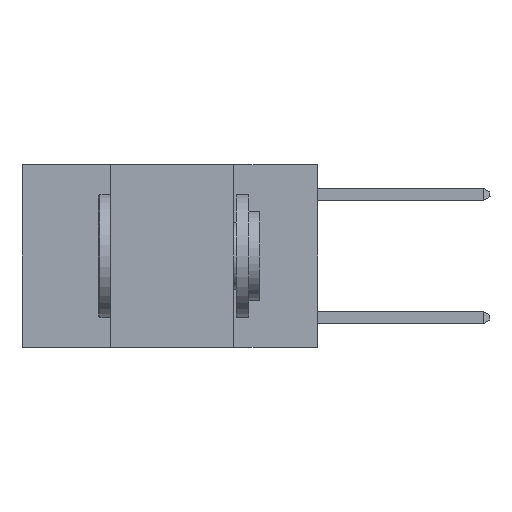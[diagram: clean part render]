
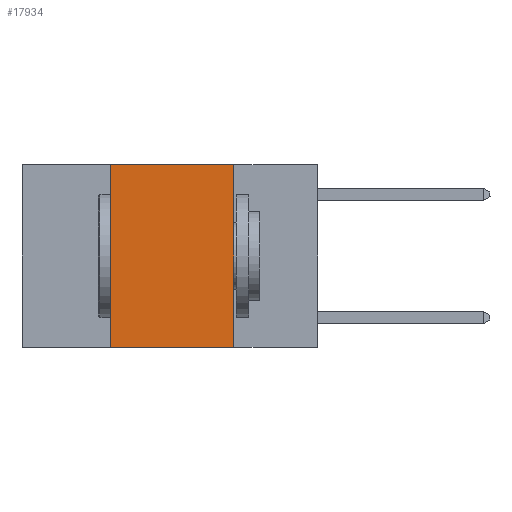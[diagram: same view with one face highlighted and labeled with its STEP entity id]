
A CAD part, left-side view. The second image highlights one B-rep face of the part: STEP entity #17934.
In plain terms, the highlighted planar face has unit normal (-1, 0, 0).
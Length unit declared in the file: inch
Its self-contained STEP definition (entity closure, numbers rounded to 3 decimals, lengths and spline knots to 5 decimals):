
#797 = ORIENTED_EDGE ( 'NONE', *, *, #24428, .T. ) ;
#1417 = VERTEX_POINT ( 'NONE', #14738 ) ;
#2218 = EDGE_CURVE ( 'NONE', #12033, #11483, #13702, .T. ) ;
#2584 = DIRECTION ( 'NONE',  ( 1., 0., 0. ) ) ;
#2837 = VECTOR ( 'NONE', #30920, 39.37008 ) ;
#5230 = VECTOR ( 'NONE', #6433, 39.37008 ) ;
#5324 = CARTESIAN_POINT ( 'NONE',  ( 0., 0.6, -0.37 ) ) ;
#5482 = CARTESIAN_POINT ( 'NONE',  ( 0., 0.17, -0.37 ) ) ;
#6433 = DIRECTION ( 'NONE',  ( 0., -1., 0. ) ) ;
#8950 = VECTOR ( 'NONE', #29893, 39.37008 ) ;
#9730 = EDGE_CURVE ( 'NONE', #1417, #12033, #31373, .T. ) ;
#9794 = LINE ( 'NONE', #26994, #8950 ) ;
#10155 = FACE_OUTER_BOUND ( 'NONE', #29602, .T. ) ;
#11453 = CARTESIAN_POINT ( 'NONE',  ( 0., 0.42, 0. ) ) ;
#11483 = VERTEX_POINT ( 'NONE', #24585 ) ;
#12033 = VERTEX_POINT ( 'NONE', #15304 ) ;
#13237 = CARTESIAN_POINT ( 'NONE',  ( 0., 0.6, 0. ) ) ;
#13702 = LINE ( 'NONE', #13237, #2837 ) ;
#14738 = CARTESIAN_POINT ( 'NONE',  ( 0., 0.42, -0.37 ) ) ;
#14982 = DIRECTION ( 'NONE',  ( 0., 0., -1. ) ) ;
#15304 = CARTESIAN_POINT ( 'NONE',  ( 0., 0.42, 0. ) ) ;
#15607 = ORIENTED_EDGE ( 'NONE', *, *, #26885, .F. ) ;
#17934 = ADVANCED_FACE ( 'NONE', ( #10155 ), #27186, .F. ) ;
#20445 = AXIS2_PLACEMENT_3D ( 'NONE', #24642, #2584, #14982 ) ;
#21248 = DIRECTION ( 'NONE',  ( 0., 0., 1. ) ) ;
#21669 = ORIENTED_EDGE ( 'NONE', *, *, #2218, .F. ) ;
#24337 = VERTEX_POINT ( 'NONE', #5482 ) ;
#24428 = EDGE_CURVE ( 'NONE', #1417, #24337, #27356, .T. ) ;
#24585 = CARTESIAN_POINT ( 'NONE',  ( 0., 0.17, 0. ) ) ;
#24642 = CARTESIAN_POINT ( 'NONE',  ( 0., 0.6, 0. ) ) ;
#26885 = EDGE_CURVE ( 'NONE', #11483, #24337, #9794, .T. ) ;
#26994 = CARTESIAN_POINT ( 'NONE',  ( 0., 0.17, 0. ) ) ;
#26995 = VECTOR ( 'NONE', #21248, 39.37008 ) ;
#27186 = PLANE ( 'NONE',  #20445 ) ;
#27356 = LINE ( 'NONE', #5324, #5230 ) ;
#27639 = ORIENTED_EDGE ( 'NONE', *, *, #9730, .F. ) ;
#29602 = EDGE_LOOP ( 'NONE', ( #15607, #21669, #27639, #797 ) ) ;
#29893 = DIRECTION ( 'NONE',  ( 0., 0., -1. ) ) ;
#30920 = DIRECTION ( 'NONE',  ( 0., -1., 0. ) ) ;
#31373 = LINE ( 'NONE', #11453, #26995 ) ;
